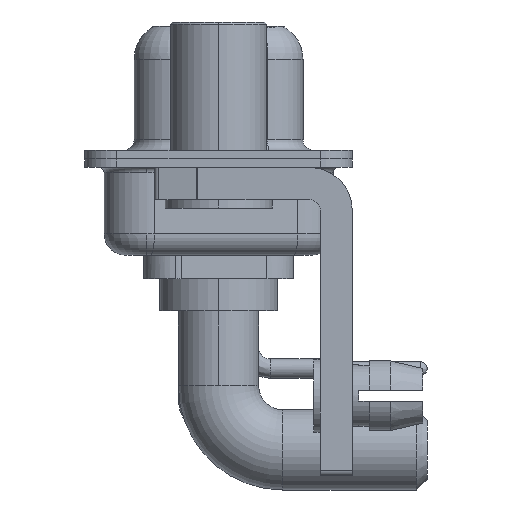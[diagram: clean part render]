
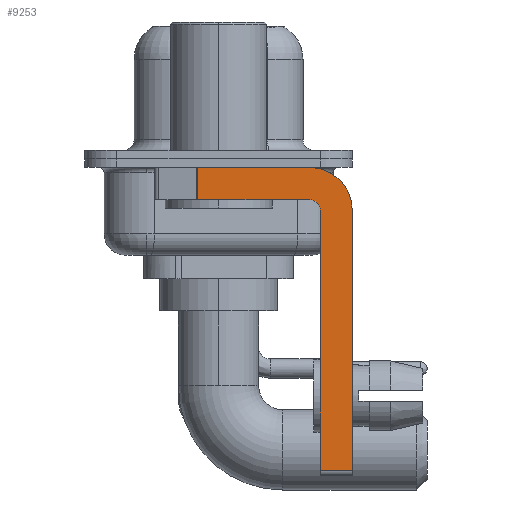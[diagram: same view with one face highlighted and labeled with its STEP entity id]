
A CAD part, left-side view. The second image highlights one B-rep face of the part: STEP entity #9253.
In plain terms, the highlighted planar face has unit normal (-1, 0, 0).
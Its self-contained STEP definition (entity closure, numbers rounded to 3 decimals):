
#214 = CARTESIAN_POINT ( 'NONE',  ( -2.9, 0.978, -1.9 ) ) ;
#215 = VERTEX_POINT ( 'NONE', #2691 ) ;
#373 = CARTESIAN_POINT ( 'NONE',  ( -2.9, -4.75, -14.55 ) ) ;
#439 = CARTESIAN_POINT ( 'NONE',  ( -2.9, -6.25, -2.4 ) ) ;
#851 = CIRCLE ( 'NONE', #23454, 2. ) ;
#936 = EDGE_CURVE ( 'NONE', #11234, #21617, #4373, .T. ) ;
#1086 = VECTOR ( 'NONE', #19940, 1000. ) ;
#1113 = CARTESIAN_POINT ( 'NONE',  ( -2.9, -4.25, -0.4 ) ) ;
#1140 = PLANE ( 'NONE',  #2777 ) ;
#1844 = EDGE_CURVE ( 'NONE', #22873, #10055, #7240, .T. ) ;
#2051 = VECTOR ( 'NONE', #20185, 1000. ) ;
#2387 = CARTESIAN_POINT ( 'NONE',  ( -2.9, -4.75, -2.4 ) ) ;
#2485 = CARTESIAN_POINT ( 'NONE',  ( -2.9, -4.75, -14.8 ) ) ;
#2562 = ORIENTED_EDGE ( 'NONE', *, *, #6906, .F. ) ;
#2619 = VERTEX_POINT ( 'NONE', #1113 ) ;
#2691 = CARTESIAN_POINT ( 'NONE',  ( -2.9, 0.978, -0.4 ) ) ;
#2777 = AXIS2_PLACEMENT_3D ( 'NONE', #8838, #12635, #2905 ) ;
#2905 = DIRECTION ( 'NONE',  ( 0., 0., -1. ) ) ;
#2957 = VECTOR ( 'NONE', #7904, 1000. ) ;
#3051 = ORIENTED_EDGE ( 'NONE', *, *, #11274, .F. ) ;
#3221 = CARTESIAN_POINT ( 'NONE',  ( -2.9, 3., -0.4 ) ) ;
#3890 = LINE ( 'NONE', #214, #20115 ) ;
#4008 = CARTESIAN_POINT ( 'NONE',  ( -2.9, -4.25, -2.4 ) ) ;
#4373 = LINE ( 'NONE', #15388, #2957 ) ;
#4524 = ORIENTED_EDGE ( 'NONE', *, *, #6828, .T. ) ;
#4538 = EDGE_LOOP ( 'NONE', ( #12414, #4524, #7465, #20359, #2562, #17583, #12721, #3051 ) ) ;
#4766 = LINE ( 'NONE', #2485, #1086 ) ;
#5468 = CARTESIAN_POINT ( 'NONE',  ( -2.9, -6.25, -2.4 ) ) ;
#5907 = DIRECTION ( 'NONE',  ( -1., 0., 0. ) ) ;
#6264 = VERTEX_POINT ( 'NONE', #373 ) ;
#6766 = CARTESIAN_POINT ( 'NONE',  ( -2.9, -4.25, -14.55 ) ) ;
#6828 = EDGE_CURVE ( 'NONE', #215, #21617, #3890, .T. ) ;
#6906 = EDGE_CURVE ( 'NONE', #6264, #15499, #4766, .T. ) ;
#7240 = LINE ( 'NONE', #5468, #17685 ) ;
#7465 = ORIENTED_EDGE ( 'NONE', *, *, #936, .F. ) ;
#7904 = DIRECTION ( 'NONE',  ( 0., 1., 0. ) ) ;
#8045 = DIRECTION ( 'NONE',  ( 0., 0., -1. ) ) ;
#8838 = CARTESIAN_POINT ( 'NONE',  ( -2.9, -4.25, -2.4 ) ) ;
#9077 = AXIS2_PLACEMENT_3D ( 'NONE', #19563, #5907, #9681 ) ;
#9253 = ADVANCED_FACE ( 'NONE', ( #20240 ), #1140, .F. ) ;
#9681 = DIRECTION ( 'NONE',  ( 0., 0., 1. ) ) ;
#10055 = VERTEX_POINT ( 'NONE', #12802 ) ;
#10709 = CIRCLE ( 'NONE', #9077, 0.5 ) ;
#10923 = DIRECTION ( 'NONE',  ( 0., -1., 0. ) ) ;
#11234 = VERTEX_POINT ( 'NONE', #16675 ) ;
#11274 = EDGE_CURVE ( 'NONE', #2619, #22873, #851, .T. ) ;
#11276 = DIRECTION ( 'NONE',  ( 0., 0., -1. ) ) ;
#12414 = ORIENTED_EDGE ( 'NONE', *, *, #12892, .F. ) ;
#12626 = EDGE_CURVE ( 'NONE', #6264, #10055, #16376, .T. ) ;
#12635 = DIRECTION ( 'NONE',  ( 1., 0., 0. ) ) ;
#12721 = ORIENTED_EDGE ( 'NONE', *, *, #1844, .F. ) ;
#12802 = CARTESIAN_POINT ( 'NONE',  ( -2.9, -6.25, -14.55 ) ) ;
#12892 = EDGE_CURVE ( 'NONE', #215, #2619, #20560, .T. ) ;
#15388 = CARTESIAN_POINT ( 'NONE',  ( -2.9, -4.25, -1.9 ) ) ;
#15499 = VERTEX_POINT ( 'NONE', #2387 ) ;
#16376 = LINE ( 'NONE', #6766, #2051 ) ;
#16675 = CARTESIAN_POINT ( 'NONE',  ( -2.9, -4.25, -1.9 ) ) ;
#17421 = DIRECTION ( 'NONE',  ( 1., 0., 0. ) ) ;
#17423 = VECTOR ( 'NONE', #10923, 1000. ) ;
#17583 = ORIENTED_EDGE ( 'NONE', *, *, #12626, .T. ) ;
#17668 = DIRECTION ( 'NONE',  ( 0., 0., -1. ) ) ;
#17685 = VECTOR ( 'NONE', #11276, 1000. ) ;
#18641 = CARTESIAN_POINT ( 'NONE',  ( -2.9, 0.978, -1.9 ) ) ;
#19546 = EDGE_CURVE ( 'NONE', #15499, #11234, #10709, .T. ) ;
#19563 = CARTESIAN_POINT ( 'NONE',  ( -2.9, -4.25, -2.4 ) ) ;
#19940 = DIRECTION ( 'NONE',  ( 0., 0., 1. ) ) ;
#20115 = VECTOR ( 'NONE', #8045, 1000. ) ;
#20185 = DIRECTION ( 'NONE',  ( 0., -1., 0. ) ) ;
#20240 = FACE_OUTER_BOUND ( 'NONE', #4538, .T. ) ;
#20359 = ORIENTED_EDGE ( 'NONE', *, *, #19546, .F. ) ;
#20560 = LINE ( 'NONE', #3221, #17423 ) ;
#21617 = VERTEX_POINT ( 'NONE', #18641 ) ;
#22873 = VERTEX_POINT ( 'NONE', #439 ) ;
#23454 = AXIS2_PLACEMENT_3D ( 'NONE', #4008, #17421, #17668 ) ;
